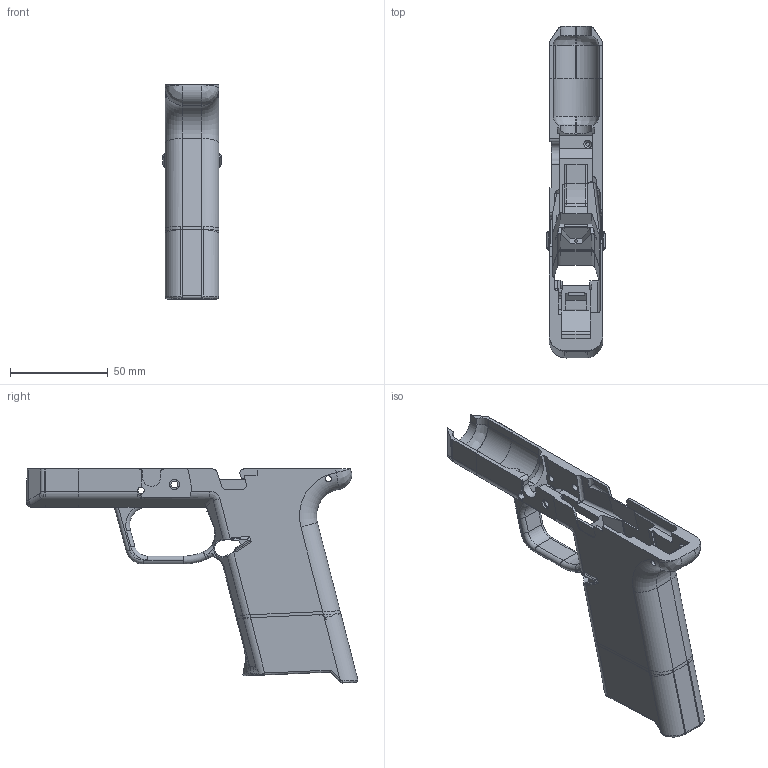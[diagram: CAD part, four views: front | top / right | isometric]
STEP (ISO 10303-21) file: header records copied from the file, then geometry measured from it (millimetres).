
FILE_DESCRIPTION(/* description */ (''),/* implementation_level */ '2;1');
FILE_NAME(/* name */ 'M&P 9 Assembly.step',/* time_stamp */ '2022-02-13T17:45:42-05:00',/* author */ (''),/* organization */ (''),/* preprocessor_version */ 'ST-DEVELOPER v18.1',/* originating_system */ 'Autodesk Translation Framework v10.13.0.1454',/* authorisation */ '');
FILE_SCHEMA (('AUTOMOTIVE_DESIGN { 1 0 10303 214 3 1 1 }','PROCESS_PLANNING_SCHEMA'));
Length unit declared in the file: millimetre
Products named in the file (6): M&P 9 Reference; Frame; Trigger Guard and Magwell; Fitment Section; M1.0 Full-size Nose; Full-Size Magwell Body
Assembly tree (5 placements, depth 4):
  M&P 9 Reference
    Frame
      Trigger Guard and Magwell
      Fitment Section
        M1.0 Full-size Nose
      Full-Size Magwell Body
Bounding box: 29.75 x 169.78 x 109.57 mm (x, y, z)
Volume: 91013.5 mm3; surface area: 49391.5 mm2
Topology: 5 solids, 5 shells, 509 faces, 1398 edges, 878 vertices
Faces by surface type: plane 218, cylinder 161, bspline 104, torus 20, sphere 4, cone 2
Full cylindrical faces by diameter (mm): 1.5 x3, 3.18 x2, 3.361 x2, 3.55 x2, 5.1 x1
Entity records: 19635 total; most frequent: CARTESIAN_POINT 6927, ORIENTED_EDGE 2774, DIRECTION 2462, EDGE_CURVE 1387, VERTEX_POINT 878, AXIS2_PLACEMENT_3D 852, LINE 758, VECTOR 758
